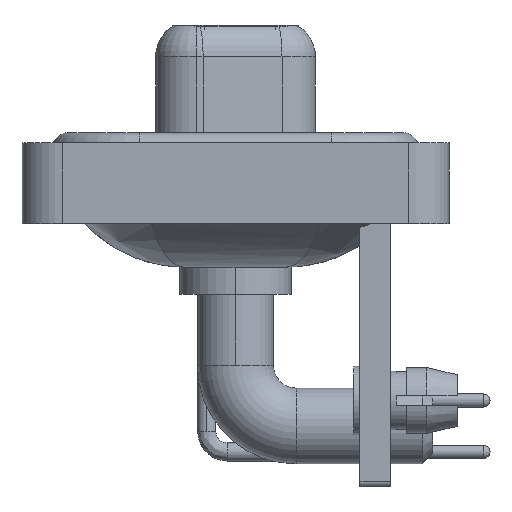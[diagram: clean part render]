
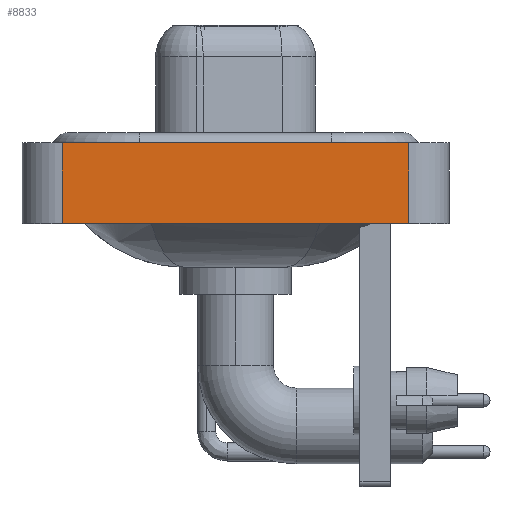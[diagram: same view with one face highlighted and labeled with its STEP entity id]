
A CAD part, left-side view. The second image highlights one B-rep face of the part: STEP entity #8833.
In plain terms, the highlighted planar face has unit normal (-1, 0, 0).
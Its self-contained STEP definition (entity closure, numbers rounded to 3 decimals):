
#377 = LINE ( 'NONE', #12382, #18532 ) ;
#382 = DIRECTION ( 'NONE',  ( 0., 0., 1. ) ) ;
#2129 = LINE ( 'NONE', #10968, #12129 ) ;
#2614 = ORIENTED_EDGE ( 'NONE', *, *, #13706, .F. ) ;
#2959 = VERTEX_POINT ( 'NONE', #10214 ) ;
#3465 = DIRECTION ( 'NONE',  ( 0., -1., 0. ) ) ;
#3675 = CARTESIAN_POINT ( 'NONE',  ( -7.3, 8.55, 0.4 ) ) ;
#3894 = VECTOR ( 'NONE', #6570, 1000. ) ;
#3964 = CARTESIAN_POINT ( 'NONE',  ( -7.3, 8.55, -3.6 ) ) ;
#3994 = DIRECTION ( 'NONE',  ( -1., 0., 0. ) ) ;
#4844 = ORIENTED_EDGE ( 'NONE', *, *, #14411, .T. ) ;
#5589 = CARTESIAN_POINT ( 'NONE',  ( -7.3, -8.55, -3.6 ) ) ;
#5741 = CARTESIAN_POINT ( 'NONE',  ( -7.3, -8.55, -3.6 ) ) ;
#6570 = DIRECTION ( 'NONE',  ( 0., 0., 1. ) ) ;
#7745 = ORIENTED_EDGE ( 'NONE', *, *, #17729, .T. ) ;
#8833 = ADVANCED_FACE ( 'NONE', ( #21643 ), #12515, .T. ) ;
#9226 = DIRECTION ( 'NONE',  ( 0., 0., 1. ) ) ;
#10214 = CARTESIAN_POINT ( 'NONE',  ( -7.3, -8.55, 0.4 ) ) ;
#10746 = EDGE_LOOP ( 'NONE', ( #4844, #17543, #2614, #7745 ) ) ;
#10968 = CARTESIAN_POINT ( 'NONE',  ( -7.3, -8.55, -3.6 ) ) ;
#11840 = CARTESIAN_POINT ( 'NONE',  ( -7.3, 8.55, -3.6 ) ) ;
#12129 = VECTOR ( 'NONE', #382, 1000. ) ;
#12199 = VERTEX_POINT ( 'NONE', #3964 ) ;
#12382 = CARTESIAN_POINT ( 'NONE',  ( -7.3, -8.55, -3.6 ) ) ;
#12515 = PLANE ( 'NONE',  #15993 ) ;
#12728 = DIRECTION ( 'NONE',  ( 0., -1., 0. ) ) ;
#13364 = EDGE_CURVE ( 'NONE', #15094, #2959, #22966, .T. ) ;
#13706 = EDGE_CURVE ( 'NONE', #12199, #15094, #17001, .T. ) ;
#14411 = EDGE_CURVE ( 'NONE', #15583, #2959, #2129, .T. ) ;
#15094 = VERTEX_POINT ( 'NONE', #3675 ) ;
#15583 = VERTEX_POINT ( 'NONE', #5589 ) ;
#15993 = AXIS2_PLACEMENT_3D ( 'NONE', #5741, #3994, #9226 ) ;
#17001 = LINE ( 'NONE', #11840, #3894 ) ;
#17113 = VECTOR ( 'NONE', #3465, 1000. ) ;
#17543 = ORIENTED_EDGE ( 'NONE', *, *, #13364, .F. ) ;
#17729 = EDGE_CURVE ( 'NONE', #12199, #15583, #377, .T. ) ;
#18532 = VECTOR ( 'NONE', #12728, 1000. ) ;
#21334 = CARTESIAN_POINT ( 'NONE',  ( -7.3, -8.55, 0.4 ) ) ;
#21643 = FACE_OUTER_BOUND ( 'NONE', #10746, .T. ) ;
#22966 = LINE ( 'NONE', #21334, #17113 ) ;
